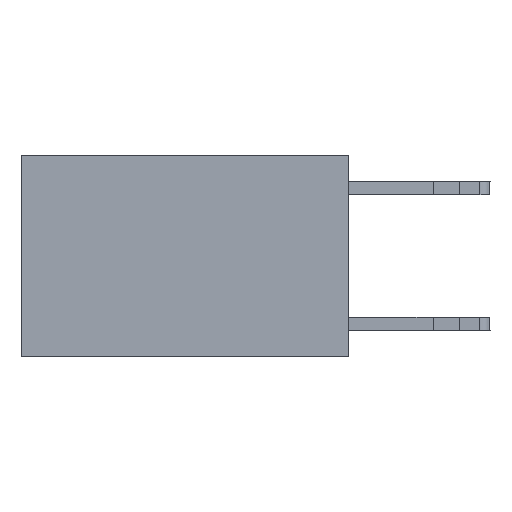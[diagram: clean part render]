
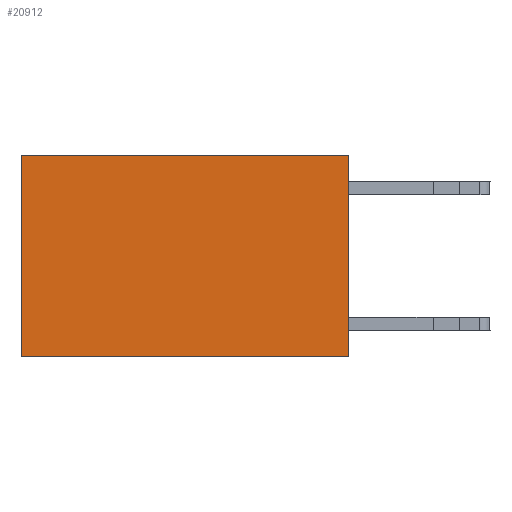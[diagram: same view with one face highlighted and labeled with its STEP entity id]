
A CAD part, left-side view. The second image highlights one B-rep face of the part: STEP entity #20912.
In plain terms, the highlighted planar face has unit normal (-1, 0, 0).
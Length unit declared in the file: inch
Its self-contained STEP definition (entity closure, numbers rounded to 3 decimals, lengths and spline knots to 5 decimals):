
#440 = EDGE_CURVE ( 'NONE', #10500, #7752, #12982, .T. ) ;
#1526 = ORIENTED_EDGE ( 'NONE', *, *, #440, .F. ) ;
#1760 = FACE_OUTER_BOUND ( 'NONE', #18480, .T. ) ;
#1842 = VERTEX_POINT ( 'NONE', #10907 ) ;
#3261 = CARTESIAN_POINT ( 'NONE',  ( 0.2625, 0., -0.37 ) ) ;
#3521 = PLANE ( 'NONE',  #9624 ) ;
#4905 = DIRECTION ( 'NONE',  ( 0., 0., -1. ) ) ;
#5023 = CARTESIAN_POINT ( 'NONE',  ( 0.2625, 0., 0. ) ) ;
#5146 = DIRECTION ( 'NONE',  ( 0., 1., 0. ) ) ;
#5343 = CARTESIAN_POINT ( 'NONE',  ( 0.2625, 0.6, 0. ) ) ;
#5474 = CARTESIAN_POINT ( 'NONE',  ( 0.2625, 0., -0.37 ) ) ;
#6392 = LINE ( 'NONE', #9888, #12268 ) ;
#6847 = VECTOR ( 'NONE', #5146, 39.37008 ) ;
#7733 = EDGE_CURVE ( 'NONE', #13102, #1842, #23416, .T. ) ;
#7752 = VERTEX_POINT ( 'NONE', #5474 ) ;
#8221 = ORIENTED_EDGE ( 'NONE', *, *, #15498, .T. ) ;
#8240 = DIRECTION ( 'NONE',  ( 0., 1., 0. ) ) ;
#9624 = AXIS2_PLACEMENT_3D ( 'NONE', #24335, #16647, #14673 ) ;
#9888 = CARTESIAN_POINT ( 'NONE',  ( 0.2625, 0., 0. ) ) ;
#10500 = VERTEX_POINT ( 'NONE', #5023 ) ;
#10907 = CARTESIAN_POINT ( 'NONE',  ( 0.2625, 0.6, -0.37 ) ) ;
#10940 = CARTESIAN_POINT ( 'NONE',  ( 0.2625, 0.6, 0. ) ) ;
#12087 = VECTOR ( 'NONE', #13738, 39.37008 ) ;
#12268 = VECTOR ( 'NONE', #8240, 39.37008 ) ;
#12982 = LINE ( 'NONE', #20542, #19692 ) ;
#13102 = VERTEX_POINT ( 'NONE', #10940 ) ;
#13738 = DIRECTION ( 'NONE',  ( 0., 0., -1. ) ) ;
#14673 = DIRECTION ( 'NONE',  ( 0., 0., -1. ) ) ;
#15498 = EDGE_CURVE ( 'NONE', #10500, #13102, #6392, .T. ) ;
#16647 = DIRECTION ( 'NONE',  ( 1., 0., 0. ) ) ;
#16892 = LINE ( 'NONE', #3261, #6847 ) ;
#16922 = ORIENTED_EDGE ( 'NONE', *, *, #20992, .F. ) ;
#18480 = EDGE_LOOP ( 'NONE', ( #23517, #16922, #1526, #8221 ) ) ;
#19692 = VECTOR ( 'NONE', #4905, 39.37008 ) ;
#20542 = CARTESIAN_POINT ( 'NONE',  ( 0.2625, 0., 0. ) ) ;
#20912 = ADVANCED_FACE ( 'NONE', ( #1760 ), #3521, .F. ) ;
#20992 = EDGE_CURVE ( 'NONE', #7752, #1842, #16892, .T. ) ;
#23416 = LINE ( 'NONE', #5343, #12087 ) ;
#23517 = ORIENTED_EDGE ( 'NONE', *, *, #7733, .T. ) ;
#24335 = CARTESIAN_POINT ( 'NONE',  ( 0.2625, 0., 0. ) ) ;
